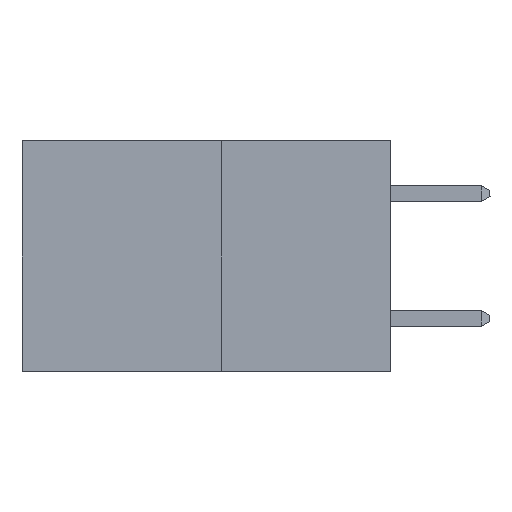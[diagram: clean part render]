
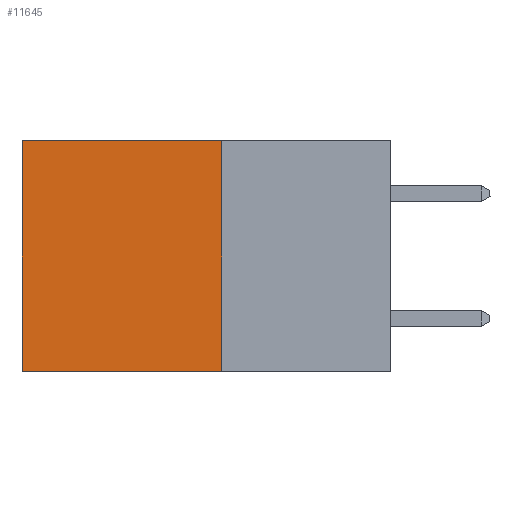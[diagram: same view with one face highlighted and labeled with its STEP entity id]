
A CAD part, left-side view. The second image highlights one B-rep face of the part: STEP entity #11645.
In plain terms, the highlighted planar face has unit normal (-1, 0, 0).
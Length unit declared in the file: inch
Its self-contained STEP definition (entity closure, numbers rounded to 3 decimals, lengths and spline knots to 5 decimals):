
#3 = EDGE_CURVE ( 'NONE', #16782, #16574, #7867, .T. ) ;
#151 = ORIENTED_EDGE ( 'NONE', *, *, #20614, .F. ) ;
#1143 = CARTESIAN_POINT ( 'NONE',  ( 0.277, 0.59, -0.37 ) ) ;
#2676 = DIRECTION ( 'NONE',  ( 0., 1., 0. ) ) ;
#2720 = DIRECTION ( 'NONE',  ( 1., 0., 0. ) ) ;
#3342 = LINE ( 'NONE', #20390, #20264 ) ;
#3482 = VECTOR ( 'NONE', #7315, 39.37008 ) ;
#3683 = VERTEX_POINT ( 'NONE', #18245 ) ;
#4110 = VECTOR ( 'NONE', #20187, 39.37008 ) ;
#4736 = ORIENTED_EDGE ( 'NONE', *, *, #10914, .T. ) ;
#5862 = VECTOR ( 'NONE', #2676, 39.37008 ) ;
#7315 = DIRECTION ( 'NONE',  ( 0., 0., -1. ) ) ;
#7808 = CARTESIAN_POINT ( 'NONE',  ( 0.277, 0.59, -0.37 ) ) ;
#7867 = LINE ( 'NONE', #7808, #3482 ) ;
#8532 = EDGE_CURVE ( 'NONE', #3683, #16574, #16693, .T. ) ;
#8754 = CARTESIAN_POINT ( 'NONE',  ( 0.277, 0.27, -0.37 ) ) ;
#10210 = LINE ( 'NONE', #12523, #5862 ) ;
#10914 = EDGE_CURVE ( 'NONE', #14795, #16782, #10210, .T. ) ;
#11380 = AXIS2_PLACEMENT_3D ( 'NONE', #19051, #2720, #14196 ) ;
#11645 = ADVANCED_FACE ( 'NONE', ( #14549 ), #12563, .F. ) ;
#12523 = CARTESIAN_POINT ( 'NONE',  ( 0.277, 0.27, 0. ) ) ;
#12563 = PLANE ( 'NONE',  #11380 ) ;
#14196 = DIRECTION ( 'NONE',  ( 0., 0., -1. ) ) ;
#14549 = FACE_OUTER_BOUND ( 'NONE', #19349, .T. ) ;
#14795 = VERTEX_POINT ( 'NONE', #19010 ) ;
#15896 = ORIENTED_EDGE ( 'NONE', *, *, #3, .T. ) ;
#16574 = VERTEX_POINT ( 'NONE', #1143 ) ;
#16693 = LINE ( 'NONE', #8754, #4110 ) ;
#16782 = VERTEX_POINT ( 'NONE', #18077 ) ;
#17181 = DIRECTION ( 'NONE',  ( 0., 0., -1. ) ) ;
#18077 = CARTESIAN_POINT ( 'NONE',  ( 0.277, 0.59, 0. ) ) ;
#18245 = CARTESIAN_POINT ( 'NONE',  ( 0.277, 0.27, -0.37 ) ) ;
#19010 = CARTESIAN_POINT ( 'NONE',  ( 0.277, 0.27, 0. ) ) ;
#19051 = CARTESIAN_POINT ( 'NONE',  ( 0.277, 0.27, -0.37 ) ) ;
#19349 = EDGE_LOOP ( 'NONE', ( #15896, #20211, #151, #4736 ) ) ;
#20187 = DIRECTION ( 'NONE',  ( 0., 1., 0. ) ) ;
#20211 = ORIENTED_EDGE ( 'NONE', *, *, #8532, .F. ) ;
#20264 = VECTOR ( 'NONE', #17181, 39.37008 ) ;
#20390 = CARTESIAN_POINT ( 'NONE',  ( 0.277, 0.27, -0.37 ) ) ;
#20614 = EDGE_CURVE ( 'NONE', #14795, #3683, #3342, .T. ) ;
